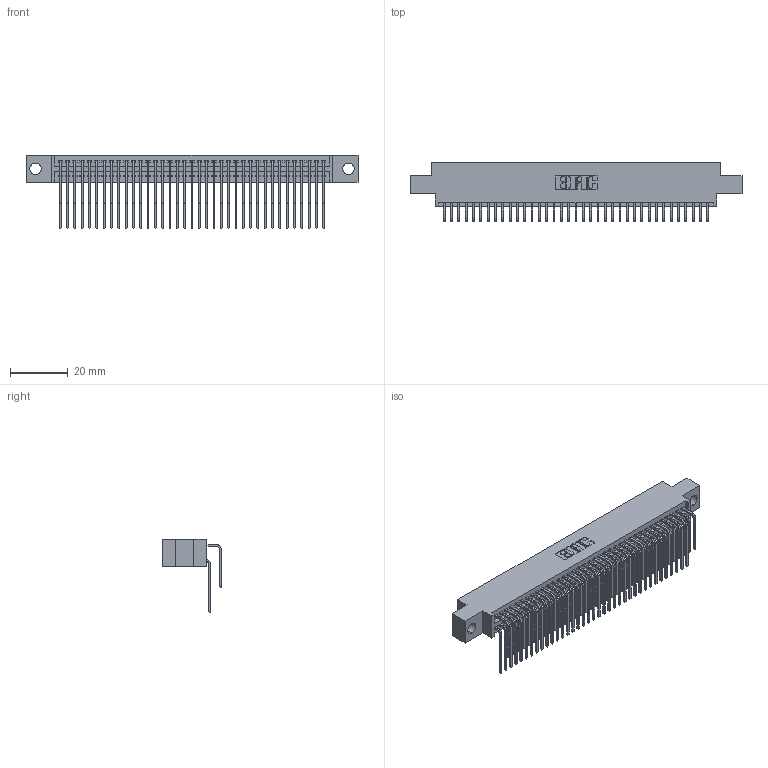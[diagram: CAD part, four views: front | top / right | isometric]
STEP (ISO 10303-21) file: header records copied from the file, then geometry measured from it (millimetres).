
FILE_DESCRIPTION (( 'STEP AP203' ), '1' );
FILE_NAME ('395-074-559-804.STEP', '2021-06-17T05:46:46', ( '' ), ( '' ), 'SwSTEP 2.0', 'SolidWorks 2020', '' );
FILE_SCHEMA (( 'CONFIG_CONTROL_DESIGN' ));
Length unit declared in the file: inch
Products named in the file (4): 345-292-001_559 Tail - 2; 345-292-001_558 559 Tail - 1; 395-074-559-804; 345 Part_0.170 Offset - 0.156 Dia-TI
Assembly tree (75 placements, depth 2):
  395-074-559-804
    345 Part_0.170 Offset - 0.156 Dia-TI
    345-292-001_558 559 Tail - 1  x37
    345-292-001_559 Tail - 2  x37
Bounding box: 115.19 x 20.56 x 25.53 mm (x, y, z)
Volume: 11350.7 mm3; surface area: 18683.9 mm2
Topology: 75 solids, 75 shells, 3992 faces, 11859 edges, 7806 vertices
Faces by surface type: plane 2688, cylinder 1304
Entity records: 31907 total; most frequent: CARTESIAN_POINT 5405, ORIENTED_EDGE 5286, DIRECTION 4743, EDGE_CURVE 2643, LINE 2323, VECTOR 2323, VERTEX_POINT 1758, AXIS2_PLACEMENT_3D 1210
